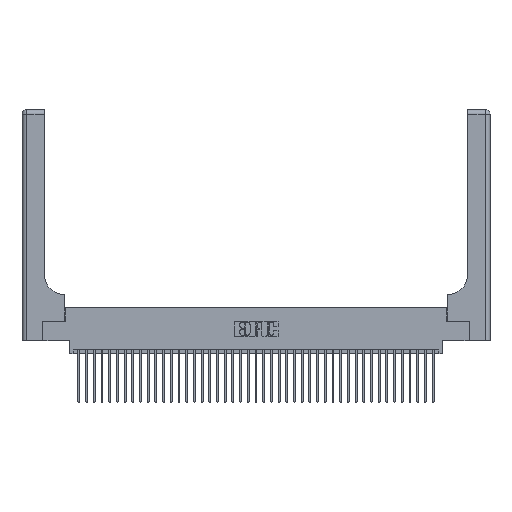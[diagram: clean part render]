
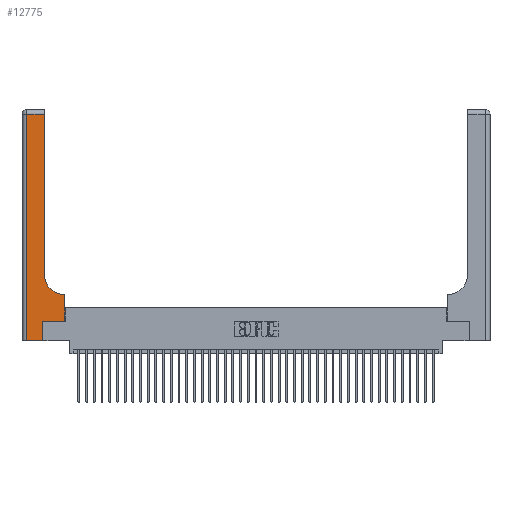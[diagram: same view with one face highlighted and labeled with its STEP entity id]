
A CAD part, top view. The second image highlights one B-rep face of the part: STEP entity #12775.
In plain terms, the highlighted planar face has unit normal (0, 0, 1).
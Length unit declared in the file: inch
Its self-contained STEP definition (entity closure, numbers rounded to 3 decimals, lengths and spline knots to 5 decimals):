
#390 = DIRECTION ( 'NONE',  ( 1., 0., 0. ) ) ;
#2642 = VECTOR ( 'NONE', #9730, 39.37008 ) ;
#4396 = EDGE_CURVE ( 'NONE', #29354, #30842, #13096, .T. ) ;
#5876 = EDGE_CURVE ( 'NONE', #30842, #24243, #12555, .T. ) ;
#6418 = CARTESIAN_POINT ( 'NONE',  ( 0.06, 3., 0.37 ) ) ;
#7417 = LINE ( 'NONE', #6418, #25565 ) ;
#7552 = VERTEX_POINT ( 'NONE', #35041 ) ;
#7795 = EDGE_CURVE ( 'NONE', #17870, #7552, #11343, .T. ) ;
#8063 = DIRECTION ( 'NONE',  ( 1., 0., 0. ) ) ;
#8354 = CARTESIAN_POINT ( 'NONE',  ( 0.5415, 0.85, 0.37 ) ) ;
#8485 = DIRECTION ( 'NONE',  ( 0., 1., 0. ) ) ;
#8566 = LINE ( 'NONE', #19980, #41472 ) ;
#8717 = CARTESIAN_POINT ( 'NONE',  ( 0., 2.94, 0.37 ) ) ;
#9090 = AXIS2_PLACEMENT_3D ( 'NONE', #31958, #16123, #38368 ) ;
#9730 = DIRECTION ( 'NONE',  ( 0., 1., 0. ) ) ;
#10013 = ORIENTED_EDGE ( 'NONE', *, *, #4396, .T. ) ;
#10366 = LINE ( 'NONE', #24115, #17954 ) ;
#11088 = LINE ( 'NONE', #38624, #26148 ) ;
#11343 = LINE ( 'NONE', #25719, #2642 ) ;
#11549 = CARTESIAN_POINT ( 'NONE',  ( 0.2915, 2.94, 0.37 ) ) ;
#11602 = DIRECTION ( 'NONE',  ( 1., 0., 0. ) ) ;
#12555 = LINE ( 'NONE', #13611, #37022 ) ;
#12775 = ADVANCED_FACE ( 'NONE', ( #37396 ), #12844, .F. ) ;
#12844 = PLANE ( 'NONE',  #9090 ) ;
#13096 = CIRCLE ( 'NONE', #16995, 0.25 ) ;
#13596 = VERTEX_POINT ( 'NONE', #26101 ) ;
#13611 = CARTESIAN_POINT ( 'NONE',  ( 0.2915, 3., 0.37 ) ) ;
#14025 = VERTEX_POINT ( 'NONE', #24653 ) ;
#14478 = EDGE_LOOP ( 'NONE', ( #36983, #23111, #35080, #26531, #24077, #38873, #27958, #18032, #10013 ) ) ;
#16123 = DIRECTION ( 'NONE',  ( 0., 0., -1. ) ) ;
#16312 = EDGE_CURVE ( 'NONE', #14025, #13596, #11088, .T. ) ;
#16703 = EDGE_CURVE ( 'NONE', #24243, #26725, #30055, .T. ) ;
#16995 = AXIS2_PLACEMENT_3D ( 'NONE', #8354, #30721, #11602 ) ;
#17475 = EDGE_CURVE ( 'NONE', #26725, #14025, #7417, .T. ) ;
#17794 = VERTEX_POINT ( 'NONE', #30210 ) ;
#17870 = VERTEX_POINT ( 'NONE', #30762 ) ;
#17954 = VECTOR ( 'NONE', #8063, 39.37008 ) ;
#18032 = ORIENTED_EDGE ( 'NONE', *, *, #21508, .T. ) ;
#19688 = CARTESIAN_POINT ( 'NONE',  ( 0.06, 2.94, 0.37 ) ) ;
#19980 = CARTESIAN_POINT ( 'NONE',  ( 0.2915, 0.6, 0.37 ) ) ;
#20533 = EDGE_CURVE ( 'NONE', #13596, #17794, #30779, .T. ) ;
#21508 = EDGE_CURVE ( 'NONE', #7552, #29354, #8566, .T. ) ;
#22938 = CARTESIAN_POINT ( 'NONE',  ( 0.5415, 0.6, 0.37 ) ) ;
#23111 = ORIENTED_EDGE ( 'NONE', *, *, #16703, .T. ) ;
#24077 = ORIENTED_EDGE ( 'NONE', *, *, #20533, .T. ) ;
#24115 = CARTESIAN_POINT ( 'NONE',  ( 0.269, 0.25, 0.37 ) ) ;
#24243 = VERTEX_POINT ( 'NONE', #11549 ) ;
#24653 = CARTESIAN_POINT ( 'NONE',  ( 0.06, 0., 0.37 ) ) ;
#25565 = VECTOR ( 'NONE', #28867, 39.37008 ) ;
#25719 = CARTESIAN_POINT ( 'NONE',  ( 0.5585, 0.25, 0.37 ) ) ;
#26101 = CARTESIAN_POINT ( 'NONE',  ( 0.269, 0., 0.37 ) ) ;
#26148 = VECTOR ( 'NONE', #390, 39.37008 ) ;
#26508 = DIRECTION ( 'NONE',  ( 0., 1., 0. ) ) ;
#26531 = ORIENTED_EDGE ( 'NONE', *, *, #16312, .T. ) ;
#26725 = VERTEX_POINT ( 'NONE', #19688 ) ;
#27958 = ORIENTED_EDGE ( 'NONE', *, *, #7795, .T. ) ;
#28867 = DIRECTION ( 'NONE',  ( 0., -1., 0. ) ) ;
#29077 = VECTOR ( 'NONE', #34314, 39.37008 ) ;
#29354 = VERTEX_POINT ( 'NONE', #22938 ) ;
#29803 = VECTOR ( 'NONE', #8485, 39.37008 ) ;
#30055 = LINE ( 'NONE', #8717, #29077 ) ;
#30210 = CARTESIAN_POINT ( 'NONE',  ( 0.269, 0.25, 0.37 ) ) ;
#30721 = DIRECTION ( 'NONE',  ( 0., 0., -1. ) ) ;
#30762 = CARTESIAN_POINT ( 'NONE',  ( 0.5585, 0.25, 0.37 ) ) ;
#30779 = LINE ( 'NONE', #30855, #29803 ) ;
#30842 = VERTEX_POINT ( 'NONE', #40939 ) ;
#30855 = CARTESIAN_POINT ( 'NONE',  ( 0.269, 0., 0.37 ) ) ;
#31958 = CARTESIAN_POINT ( 'NONE',  ( 0., 3., 0.37 ) ) ;
#34314 = DIRECTION ( 'NONE',  ( -1., 0., 0. ) ) ;
#35041 = CARTESIAN_POINT ( 'NONE',  ( 0.5585, 0.6, 0.37 ) ) ;
#35080 = ORIENTED_EDGE ( 'NONE', *, *, #17475, .T. ) ;
#36983 = ORIENTED_EDGE ( 'NONE', *, *, #5876, .T. ) ;
#37022 = VECTOR ( 'NONE', #26508, 39.37008 ) ;
#37396 = FACE_OUTER_BOUND ( 'NONE', #14478, .T. ) ;
#38368 = DIRECTION ( 'NONE',  ( -1., 0., 0. ) ) ;
#38624 = CARTESIAN_POINT ( 'NONE',  ( 0., 0., 0.37 ) ) ;
#38873 = ORIENTED_EDGE ( 'NONE', *, *, #40455, .T. ) ;
#38977 = DIRECTION ( 'NONE',  ( -1., 0., 0. ) ) ;
#40455 = EDGE_CURVE ( 'NONE', #17794, #17870, #10366, .T. ) ;
#40939 = CARTESIAN_POINT ( 'NONE',  ( 0.2915, 0.85, 0.37 ) ) ;
#41472 = VECTOR ( 'NONE', #38977, 39.37008 ) ;
